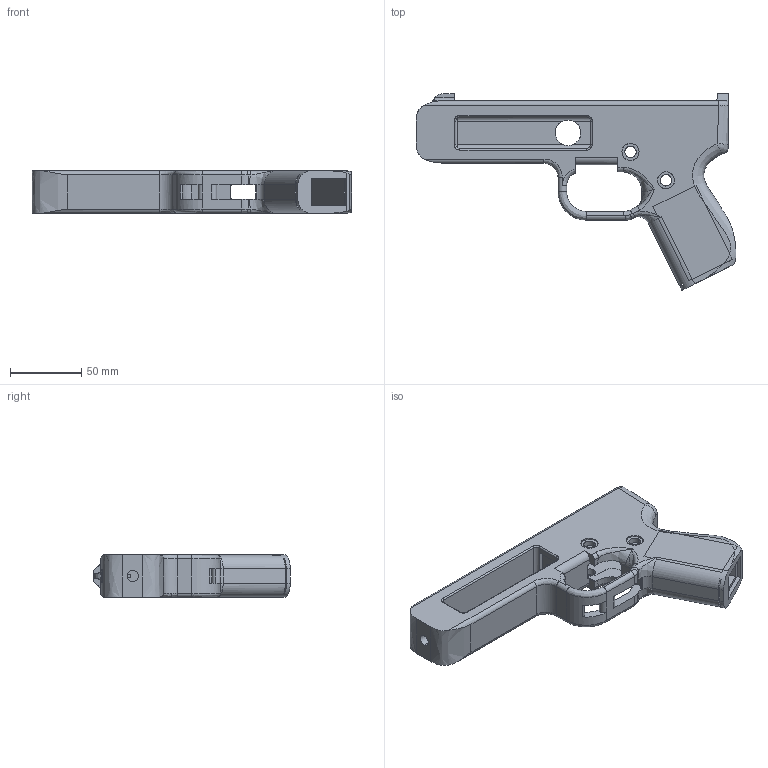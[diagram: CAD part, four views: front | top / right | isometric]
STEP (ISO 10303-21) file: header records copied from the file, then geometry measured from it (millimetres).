
FILE_DESCRIPTION(('STEP AP214'),'1');
FILE_NAME('Design2.stp','2019-06-25T13:55:24',(' '),(' '),'Spatial InterOp 3D',' ',' ');
FILE_SCHEMA(('AUTOMOTIVE_DESIGN { 1 0 10303 214 1 1 1 1 }'));
Length unit declared in the file: metre
Products named in the file (4): rahmen_legal_verbessert; Component1; Component2; Design2
Assembly tree (3 placements, depth 3):
  Design2
    rahmen_legal_verbessert
      Component1
      Component2
Bounding box: 225.28 x 138.4 x 30 mm (x, y, z)
Volume: 248231 mm3; surface area: 76236.4 mm2
Topology: 2 solids, 2 shells, 308 faces, 924 edges, 605 vertices
Faces by surface type: plane 124, cylinder 112, bspline 69, extrusion 2, torus 1
Entity records: 23855 total; most frequent: CARTESIAN_POINT 13979, ORIENTED_EDGE 1834, DIRECTION 1081, EDGE_CURVE 917, VERTEX_POINT 605, VECTOR 403, LINE 401, B_SPLINE_CURVE_WITH_KNOTS 398
